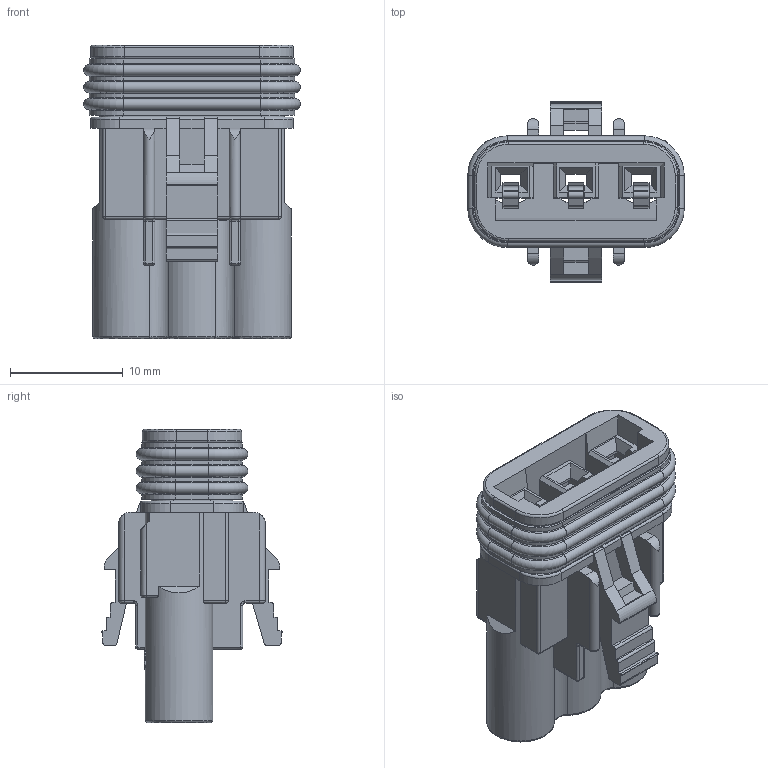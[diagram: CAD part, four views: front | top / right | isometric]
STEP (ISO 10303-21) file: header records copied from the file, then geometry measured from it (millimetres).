
FILE_DESCRIPTION (( 'STEP AP214' ), '1' );
FILE_NAME ('572-003-000-200.STEP', '2020-07-30T19:01:27', ( '' ), ( '' ), 'SwSTEP 2.0', 'SolidWorks 2020', '' );
FILE_SCHEMA (( 'AUTOMOTIVE_DESIGN' ));
Length unit declared in the file: millimetre
Products named in the file (3): 570-003-000-HOUSING-SEAL; 572-003-000-FEMALE-HOUSING_WHITE; 572-003-000-200
Assembly tree (2 placements, depth 2):
  572-003-000-200
    572-003-000-FEMALE-HOUSING_WHITE
    570-003-000-HOUSING-SEAL
Bounding box: 19.2 x 16 x 26 mm (x, y, z)
Volume: 1996.2 mm3; surface area: 4317.3 mm2
Topology: 2 solids, 4 shells, 794 faces, 2028 edges, 1232 vertices
Faces by surface type: plane 388, cylinder 257, torus 118, bspline 12, sphere 10, cone 9
Entity records: 24287 total; most frequent: CARTESIAN_POINT 5025, DIRECTION 4052, ORIENTED_EDGE 4036, EDGE_CURVE 2018, AXIS2_PLACEMENT_3D 1434, VERTEX_POINT 1232, LINE 1184, VECTOR 1184
